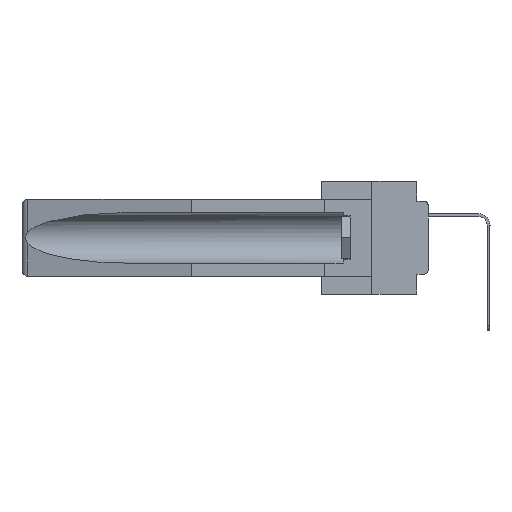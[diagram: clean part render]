
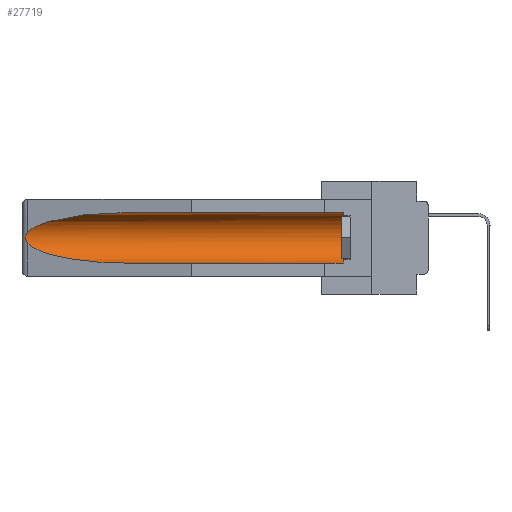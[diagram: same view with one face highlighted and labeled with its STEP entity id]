
A CAD part, left-side view. The second image highlights one B-rep face of the part: STEP entity #27719.
In plain terms, the highlighted cylindrical face has radius 2.857 mm (diameter 5.715 mm), a partial arc.
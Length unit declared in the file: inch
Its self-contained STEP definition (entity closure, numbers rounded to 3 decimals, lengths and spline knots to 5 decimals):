
#1822 = VERTEX_POINT ( 'NONE', #27605 ) ;
#1866 = CARTESIAN_POINT ( 'NONE',  ( 0.26537, 1.52718, -0.14972 ) ) ;
#2118 = CARTESIAN_POINT ( 'NONE',  ( 0.26655, 1.53094, -0.18657 ) ) ;
#2319 = CARTESIAN_POINT ( 'NONE',  ( 0.2675, 1.53308, -0.17534 ) ) ;
#2524 = CARTESIAN_POINT ( 'NONE',  ( 0.26597, 1.5296, -0.19026 ) ) ;
#2582 = CARTESIAN_POINT ( 'NONE',  ( 0.155, 1.07973, -0.284 ) ) ;
#4114 = CIRCLE ( 'NONE', #14999, 0.1125 ) ;
#4590 = CARTESIAN_POINT ( 'NONE',  ( 0.155, -0.30754, -0.059 ) ) ;
#4907 = CARTESIAN_POINT ( 'NONE',  ( 0.155, 1.07973, -0.059 ) ) ;
#5247 = VECTOR ( 'NONE', #16181, 39.37008 ) ;
#5760 = CARTESIAN_POINT ( 'NONE',  ( 0.25451, 1.48313, -0.24835 ) ) ;
#5789 = EDGE_CURVE ( 'NONE', #22098, #21037, #16994, .T. ) ;
#5840 = CARTESIAN_POINT ( 'NONE',  ( 0.155, 0.126, -0.284 ) ) ;
#6477 = ORIENTED_EDGE ( 'NONE', *, *, #10094, .F. ) ;
#7171 = ORIENTED_EDGE ( 'NONE', *, *, #24911, .T. ) ;
#7516 = VERTEX_POINT ( 'NONE', #2582 ) ;
#9573 = VERTEX_POINT ( 'NONE', #5840 ) ;
#10086 = CARTESIAN_POINT ( 'NONE',  ( 0.155, -0.30754, -0.284 ) ) ;
#10094 = EDGE_CURVE ( 'NONE', #9573, #7516, #13800, .T. ) ;
#10440 = CARTESIAN_POINT ( 'NONE',  ( 0.21114, 1.30732, -0.284 ) ) ;
#10565 = DIRECTION ( 'NONE',  ( 0., 0., 1. ) ) ;
#11136 = CARTESIAN_POINT ( 'NONE',  ( 0.155, 0.126, -0.1715 ) ) ;
#11629 = CARTESIAN_POINT ( 'NONE',  ( 0.26597, 1.52961, -0.15275 ) ) ;
#12528 = AXIS2_PLACEMENT_3D ( 'NONE', #22358, #12543, #10565 ) ;
#12543 = DIRECTION ( 'NONE',  ( 0., 1., 0. ) ) ;
#12599 = EDGE_CURVE ( 'NONE', #9573, #22098, #4114, .T. ) ;
#12760 = DIRECTION ( 'NONE',  ( 0., 1., 0. ) ) ;
#13134 = CARTESIAN_POINT ( 'NONE',  ( 0.26537, 1.52718, -0.19328 ) ) ;
#13800 = LINE ( 'NONE', #10086, #15614 ) ;
#13829 =( BOUNDED_CURVE ( )  B_SPLINE_CURVE ( 3, ( #22758, #20564, #25455, #1866 ),
 .UNSPECIFIED., .F., .F. ) 
 B_SPLINE_CURVE_WITH_KNOTS ( ( 4, 4 ),
 ( 4.71239, 6.08839 ),
 .UNSPECIFIED. ) 
 CURVE ( )  GEOMETRIC_REPRESENTATION_ITEM ( )  RATIONAL_B_SPLINE_CURVE ( ( 1., 0.848, 0.848, 1. ) ) 
 REPRESENTATION_ITEM ( '' )  );
#13843 = FACE_OUTER_BOUND ( 'NONE', #22600, .T. ) ;
#14586 = CARTESIAN_POINT ( 'NONE',  ( 0.2673, 1.5327, -0.16383 ) ) ;
#14906 = ORIENTED_EDGE ( 'NONE', *, *, #30030, .T. ) ;
#14999 = AXIS2_PLACEMENT_3D ( 'NONE', #11136, #25316, #17954 ) ;
#15614 = VECTOR ( 'NONE', #12760, 39.37008 ) ;
#16175 = CARTESIAN_POINT ( 'NONE',  ( 0.26654, 1.53092, -0.15636 ) ) ;
#16181 = DIRECTION ( 'NONE',  ( 0., 1., 0. ) ) ;
#16466 = EDGE_CURVE ( 'NONE', #24273, #1822, #16639, .T. ) ;
#16582 = CARTESIAN_POINT ( 'NONE',  ( 0.2675, 1.53308, -0.16763 ) ) ;
#16611 = ORIENTED_EDGE ( 'NONE', *, *, #12599, .T. ) ;
#16639 = B_SPLINE_CURVE_WITH_KNOTS ( 'NONE', 3,
 ( #30421, #11629, #16175, #14586, #16582, #2319, #21009, #2118, #2524, #28075 ),
 .UNSPECIFIED., .F., .F.,
 ( 4, 2, 2, 2, 4 ),
 ( 0., 0.00029, 0.00058, 0.00087, 0.00117 ),
 .UNSPECIFIED. ) ;
#16785 = CYLINDRICAL_SURFACE ( 'NONE', #12528, 0.1125 ) ;
#16994 = LINE ( 'NONE', #4590, #5247 ) ;
#17301 = ORIENTED_EDGE ( 'NONE', *, *, #16466, .T. ) ;
#17954 = DIRECTION ( 'NONE',  ( 0., 0., 1. ) ) ;
#18195 = CARTESIAN_POINT ( 'NONE',  ( 0.155, 0.126, -0.059 ) ) ;
#20564 = CARTESIAN_POINT ( 'NONE',  ( 0.21114, 1.30732, -0.059 ) ) ;
#21009 = CARTESIAN_POINT ( 'NONE',  ( 0.2673, 1.53269, -0.17917 ) ) ;
#21037 = VERTEX_POINT ( 'NONE', #4907 ) ;
#22098 = VERTEX_POINT ( 'NONE', #18195 ) ;
#22358 = CARTESIAN_POINT ( 'NONE',  ( 0.155, -0.30754, -0.1715 ) ) ;
#22600 = EDGE_LOOP ( 'NONE', ( #14906, #17301, #7171, #6477, #16611, #22917 ) ) ;
#22758 = CARTESIAN_POINT ( 'NONE',  ( 0.155, 1.07973, -0.059 ) ) ;
#22917 = ORIENTED_EDGE ( 'NONE', *, *, #5789, .T. ) ;
#23083 =( BOUNDED_CURVE ( )  B_SPLINE_CURVE ( 3, ( #13134, #5760, #10440, #29341 ),
 .UNSPECIFIED., .F., .F. ) 
 B_SPLINE_CURVE_WITH_KNOTS ( ( 4, 4 ),
 ( 0.1948, 1.5708 ),
 .UNSPECIFIED. ) 
 CURVE ( )  GEOMETRIC_REPRESENTATION_ITEM ( )  RATIONAL_B_SPLINE_CURVE ( ( 1., 0.848, 0.848, 1. ) ) 
 REPRESENTATION_ITEM ( '' )  );
#24273 = VERTEX_POINT ( 'NONE', #29376 ) ;
#24911 = EDGE_CURVE ( 'NONE', #1822, #7516, #23083, .T. ) ;
#25316 = DIRECTION ( 'NONE',  ( 0., -1., 0. ) ) ;
#25455 = CARTESIAN_POINT ( 'NONE',  ( 0.25451, 1.48313, -0.09465 ) ) ;
#27605 = CARTESIAN_POINT ( 'NONE',  ( 0.26537, 1.52718, -0.19328 ) ) ;
#27719 = ADVANCED_FACE ( 'NONE', ( #13843 ), #16785, .F. ) ;
#28075 = CARTESIAN_POINT ( 'NONE',  ( 0.26537, 1.52718, -0.19328 ) ) ;
#29341 = CARTESIAN_POINT ( 'NONE',  ( 0.155, 1.07973, -0.284 ) ) ;
#29376 = CARTESIAN_POINT ( 'NONE',  ( 0.26537, 1.52718, -0.14972 ) ) ;
#30030 = EDGE_CURVE ( 'NONE', #21037, #24273, #13829, .T. ) ;
#30421 = CARTESIAN_POINT ( 'NONE',  ( 0.26537, 1.52718, -0.14972 ) ) ;
